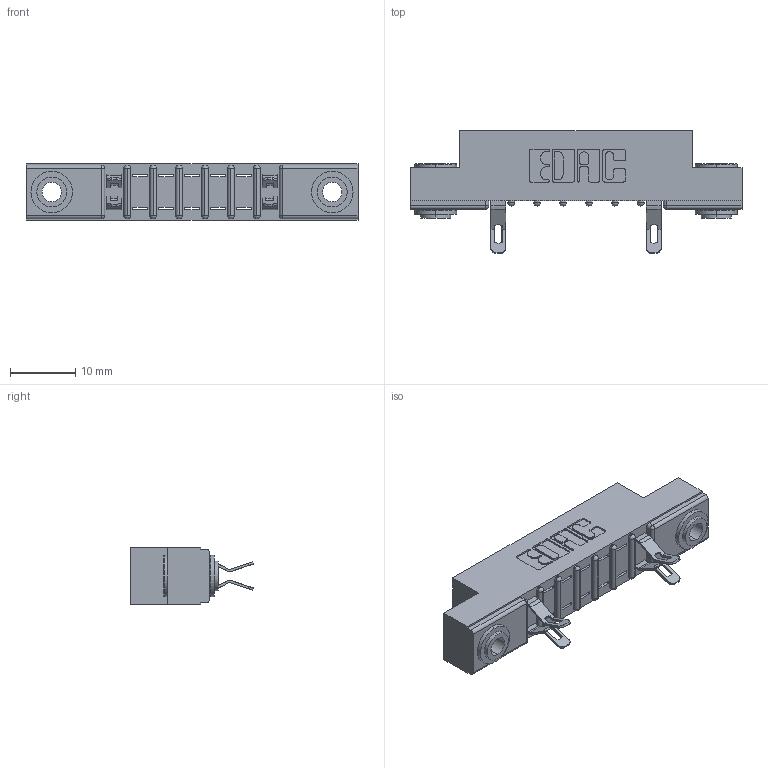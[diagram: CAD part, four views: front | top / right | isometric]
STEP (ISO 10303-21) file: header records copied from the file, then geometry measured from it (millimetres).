
FILE_DESCRIPTION (( 'STEP AP203' ), '1' );
FILE_NAME ('357-014-555-203.STEP', '2018-08-08T00:27:00', ( '' ), ( '' ), 'SwSTEP 2.0', 'SolidWorks 2016', '' );
FILE_SCHEMA (( 'CONFIG_CONTROL_DESIGN' ));
Length unit declared in the file: inch
Products named in the file (4): 307 Part_.156 Dia Mounting Holes; 307-290-001_555; 345-250-002_345-250-002-102; 357-014-555-203
Assembly tree (7 placements, depth 2):
  357-014-555-203
    307 Part_.156 Dia Mounting Holes
    307-290-001_555  x4
    345-250-002_345-250-002-102  x2
Bounding box: 50.75 x 18.75 x 8.71 mm (x, y, z)
Volume: 3205 mm3; surface area: 4427 mm2
Topology: 7 solids, 7 shells, 522 faces, 1479 edges, 954 vertices
Faces by surface type: plane 290, cylinder 208, sphere 16, cone 8
Entity records: 11822 total; most frequent: CARTESIAN_POINT 1974, DIRECTION 1960, ORIENTED_EDGE 1956, EDGE_CURVE 978, VECTOR 716, LINE 716, VERTEX_POINT 636, AXIS2_PLACEMENT_3D 622
